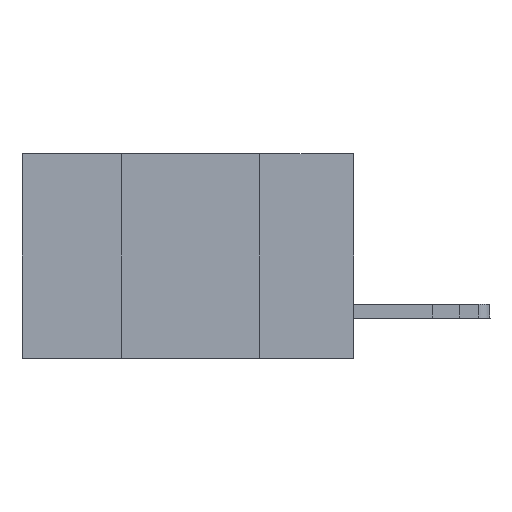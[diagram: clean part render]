
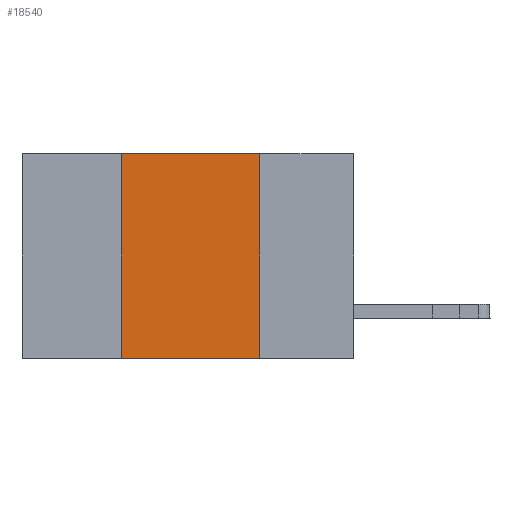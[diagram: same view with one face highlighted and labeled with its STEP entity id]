
A CAD part, left-side view. The second image highlights one B-rep face of the part: STEP entity #18540.
In plain terms, the highlighted planar face has unit normal (-1, 0, 0).
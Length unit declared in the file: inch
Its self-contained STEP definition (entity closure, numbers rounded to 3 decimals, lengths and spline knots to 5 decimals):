
#182 = CARTESIAN_POINT ( 'NONE',  ( 0., 0.42, -0.37 ) ) ;
#523 = DIRECTION ( 'NONE',  ( 1., 0., 0. ) ) ;
#3134 = EDGE_CURVE ( 'NONE', #14207, #16989, #18279, .T. ) ;
#3742 = CARTESIAN_POINT ( 'NONE',  ( 0., 0.17, 0. ) ) ;
#4070 = CARTESIAN_POINT ( 'NONE',  ( 0., 0.42, 0. ) ) ;
#4203 = CARTESIAN_POINT ( 'NONE',  ( 0., 0.42, 0. ) ) ;
#4424 = VECTOR ( 'NONE', #11205, 39.37008 ) ;
#5223 = VECTOR ( 'NONE', #18443, 39.37008 ) ;
#5234 = DIRECTION ( 'NONE',  ( 0., -1., 0. ) ) ;
#6891 = ORIENTED_EDGE ( 'NONE', *, *, #15103, .F. ) ;
#6999 = CARTESIAN_POINT ( 'NONE',  ( 0., 0.6, 0. ) ) ;
#7772 = VERTEX_POINT ( 'NONE', #4203 ) ;
#8627 = PLANE ( 'NONE',  #9539 ) ;
#9397 = LINE ( 'NONE', #4070, #13810 ) ;
#9539 = AXIS2_PLACEMENT_3D ( 'NONE', #6999, #523, #11950 ) ;
#11205 = DIRECTION ( 'NONE',  ( 0., -1., 0. ) ) ;
#11619 = FACE_OUTER_BOUND ( 'NONE', #18790, .T. ) ;
#11950 = DIRECTION ( 'NONE',  ( 0., 0., -1. ) ) ;
#12904 = CARTESIAN_POINT ( 'NONE',  ( 0., 0.17, 0. ) ) ;
#13069 = VECTOR ( 'NONE', #5234, 39.37008 ) ;
#13585 = LINE ( 'NONE', #16712, #13069 ) ;
#13806 = DIRECTION ( 'NONE',  ( 0., 0., 1. ) ) ;
#13810 = VECTOR ( 'NONE', #13806, 39.37008 ) ;
#14207 = VERTEX_POINT ( 'NONE', #12904 ) ;
#14618 = ORIENTED_EDGE ( 'NONE', *, *, #3134, .F. ) ;
#15103 = EDGE_CURVE ( 'NONE', #18384, #7772, #9397, .T. ) ;
#15622 = ORIENTED_EDGE ( 'NONE', *, *, #20610, .T. ) ;
#16712 = CARTESIAN_POINT ( 'NONE',  ( 0., 0.6, -0.37 ) ) ;
#16989 = VERTEX_POINT ( 'NONE', #17663 ) ;
#17482 = LINE ( 'NONE', #19350, #4424 ) ;
#17663 = CARTESIAN_POINT ( 'NONE',  ( 0., 0.17, -0.37 ) ) ;
#18279 = LINE ( 'NONE', #3742, #5223 ) ;
#18384 = VERTEX_POINT ( 'NONE', #182 ) ;
#18443 = DIRECTION ( 'NONE',  ( 0., 0., -1. ) ) ;
#18540 = ADVANCED_FACE ( 'NONE', ( #11619 ), #8627, .F. ) ;
#18790 = EDGE_LOOP ( 'NONE', ( #14618, #18927, #6891, #15622 ) ) ;
#18895 = EDGE_CURVE ( 'NONE', #7772, #14207, #17482, .T. ) ;
#18927 = ORIENTED_EDGE ( 'NONE', *, *, #18895, .F. ) ;
#19350 = CARTESIAN_POINT ( 'NONE',  ( 0., 0.6, 0. ) ) ;
#20610 = EDGE_CURVE ( 'NONE', #18384, #16989, #13585, .T. ) ;
